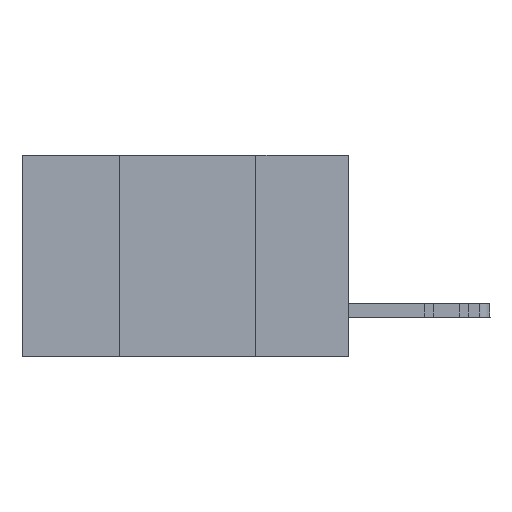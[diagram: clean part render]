
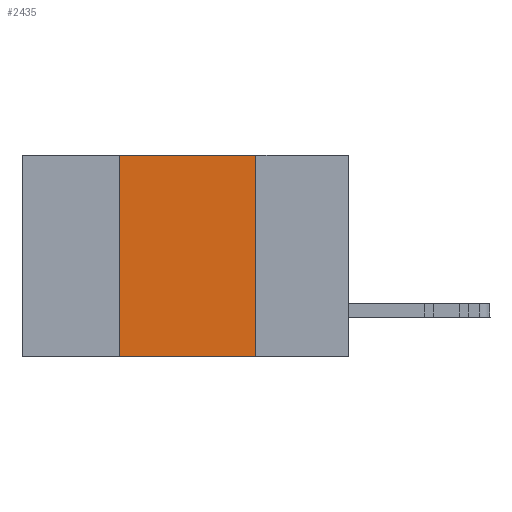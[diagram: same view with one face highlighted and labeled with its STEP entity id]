
A CAD part, left-side view. The second image highlights one B-rep face of the part: STEP entity #2435.
In plain terms, the highlighted planar face has unit normal (-1, 0, 0).
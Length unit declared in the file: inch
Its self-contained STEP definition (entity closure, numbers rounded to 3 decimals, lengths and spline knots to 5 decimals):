
#798 = CARTESIAN_POINT ( 'NONE',  ( 0., 0.6, -0.37 ) ) ;
#1250 = DIRECTION ( 'NONE',  ( 0., -1., 0. ) ) ;
#1306 = CARTESIAN_POINT ( 'NONE',  ( 0., 0.42, 0. ) ) ;
#1422 = CARTESIAN_POINT ( 'NONE',  ( 0., 0.17, 0. ) ) ;
#2408 = FACE_OUTER_BOUND ( 'NONE', #24739, .T. ) ;
#2435 = ADVANCED_FACE ( 'NONE', ( #2408 ), #9698, .F. ) ;
#2589 = ORIENTED_EDGE ( 'NONE', *, *, #12317, .F. ) ;
#3165 = CARTESIAN_POINT ( 'NONE',  ( 0., 0.42, -0.37 ) ) ;
#3613 = LINE ( 'NONE', #1306, #11209 ) ;
#4830 = VECTOR ( 'NONE', #1250, 39.37008 ) ;
#9065 = VECTOR ( 'NONE', #16849, 39.37008 ) ;
#9698 = PLANE ( 'NONE',  #19156 ) ;
#11209 = VECTOR ( 'NONE', #26740, 39.37008 ) ;
#12317 = EDGE_CURVE ( 'NONE', #23892, #21150, #18475, .T. ) ;
#13171 = CARTESIAN_POINT ( 'NONE',  ( 0., 0.17, 0. ) ) ;
#13783 = EDGE_CURVE ( 'NONE', #17300, #21150, #22100, .T. ) ;
#13838 = CARTESIAN_POINT ( 'NONE',  ( 0., 0.6, 0. ) ) ;
#14602 = VERTEX_POINT ( 'NONE', #25235 ) ;
#14847 = ORIENTED_EDGE ( 'NONE', *, *, #19770, .F. ) ;
#14943 = EDGE_CURVE ( 'NONE', #17300, #14602, #3613, .T. ) ;
#16849 = DIRECTION ( 'NONE',  ( 0., -1., 0. ) ) ;
#17300 = VERTEX_POINT ( 'NONE', #3165 ) ;
#18475 = LINE ( 'NONE', #13171, #29064 ) ;
#19114 = LINE ( 'NONE', #27812, #9065 ) ;
#19156 = AXIS2_PLACEMENT_3D ( 'NONE', #13838, #25837, #20980 ) ;
#19770 = EDGE_CURVE ( 'NONE', #14602, #23892, #19114, .T. ) ;
#20980 = DIRECTION ( 'NONE',  ( 0., 0., -1. ) ) ;
#21150 = VERTEX_POINT ( 'NONE', #28546 ) ;
#22100 = LINE ( 'NONE', #798, #4830 ) ;
#23892 = VERTEX_POINT ( 'NONE', #1422 ) ;
#24739 = EDGE_LOOP ( 'NONE', ( #2589, #14847, #25143, #29544 ) ) ;
#25143 = ORIENTED_EDGE ( 'NONE', *, *, #14943, .F. ) ;
#25235 = CARTESIAN_POINT ( 'NONE',  ( 0., 0.42, 0. ) ) ;
#25837 = DIRECTION ( 'NONE',  ( 1., 0., 0. ) ) ;
#26740 = DIRECTION ( 'NONE',  ( 0., 0., 1. ) ) ;
#27303 = DIRECTION ( 'NONE',  ( 0., 0., -1. ) ) ;
#27812 = CARTESIAN_POINT ( 'NONE',  ( 0., 0.6, 0. ) ) ;
#28546 = CARTESIAN_POINT ( 'NONE',  ( 0., 0.17, -0.37 ) ) ;
#29064 = VECTOR ( 'NONE', #27303, 39.37008 ) ;
#29544 = ORIENTED_EDGE ( 'NONE', *, *, #13783, .T. ) ;
